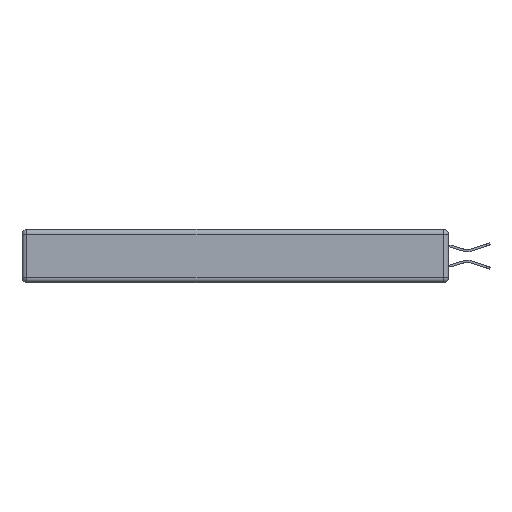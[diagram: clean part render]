
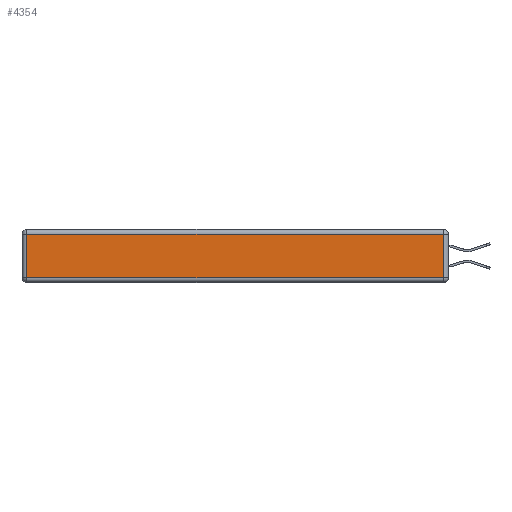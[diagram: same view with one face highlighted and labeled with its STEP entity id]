
A CAD part, left-side view. The second image highlights one B-rep face of the part: STEP entity #4354.
In plain terms, the highlighted planar face has unit normal (-1, 0, 0).
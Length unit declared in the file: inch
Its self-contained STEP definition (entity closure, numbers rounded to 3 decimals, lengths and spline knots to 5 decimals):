
#211 = FACE_OUTER_BOUND ( 'NONE', #3183, .T. ) ;
#361 = VERTEX_POINT ( 'NONE', #15520 ) ;
#588 = VERTEX_POINT ( 'NONE', #12905 ) ;
#858 = LINE ( 'NONE', #8978, #6349 ) ;
#1086 = DIRECTION ( 'NONE',  ( -1., 0., 0. ) ) ;
#1847 = DIRECTION ( 'NONE',  ( 0., 0., -1. ) ) ;
#2959 = AXIS2_PLACEMENT_3D ( 'NONE', #13436, #1086, #5044 ) ;
#3183 = EDGE_LOOP ( 'NONE', ( #13286, #7519, #15727, #15688 ) ) ;
#3670 = EDGE_CURVE ( 'NONE', #4537, #588, #15774, .T. ) ;
#4354 = ADVANCED_FACE ( 'NONE', ( #211 ), #10947, .T. ) ;
#4537 = VERTEX_POINT ( 'NONE', #11445 ) ;
#5044 = DIRECTION ( 'NONE',  ( 0., 0., 1. ) ) ;
#6349 = VECTOR ( 'NONE', #9141, 39.37008 ) ;
#7519 = ORIENTED_EDGE ( 'NONE', *, *, #15940, .T. ) ;
#7658 = EDGE_CURVE ( 'NONE', #361, #4537, #9365, .T. ) ;
#8339 = EDGE_CURVE ( 'NONE', #13849, #361, #8760, .T. ) ;
#8760 = LINE ( 'NONE', #9498, #12446 ) ;
#8972 = VECTOR ( 'NONE', #1847, 39.37008 ) ;
#8978 = CARTESIAN_POINT ( 'NONE',  ( 0., 0.03, -0.343 ) ) ;
#9141 = DIRECTION ( 'NONE',  ( 0., 0., 1. ) ) ;
#9365 = LINE ( 'NONE', #11850, #8972 ) ;
#9498 = CARTESIAN_POINT ( 'NONE',  ( 0., 2.75, -0.03 ) ) ;
#9984 = DIRECTION ( 'NONE',  ( 0., 1., 0. ) ) ;
#10947 = PLANE ( 'NONE',  #2959 ) ;
#11445 = CARTESIAN_POINT ( 'NONE',  ( 0., 2.72, -0.313 ) ) ;
#11850 = CARTESIAN_POINT ( 'NONE',  ( 0., 2.72, -0.343 ) ) ;
#12446 = VECTOR ( 'NONE', #9984, 39.37008 ) ;
#12816 = CARTESIAN_POINT ( 'NONE',  ( 0., 0., -0.313 ) ) ;
#12858 = CARTESIAN_POINT ( 'NONE',  ( 0., 0.03, -0.03 ) ) ;
#12905 = CARTESIAN_POINT ( 'NONE',  ( 0., 0.03, -0.313 ) ) ;
#13286 = ORIENTED_EDGE ( 'NONE', *, *, #3670, .T. ) ;
#13436 = CARTESIAN_POINT ( 'NONE',  ( 0., 0., -0.343 ) ) ;
#13849 = VERTEX_POINT ( 'NONE', #12858 ) ;
#13984 = DIRECTION ( 'NONE',  ( 0., -1., 0. ) ) ;
#14418 = VECTOR ( 'NONE', #13984, 39.37008 ) ;
#15520 = CARTESIAN_POINT ( 'NONE',  ( 0., 2.72, -0.03 ) ) ;
#15688 = ORIENTED_EDGE ( 'NONE', *, *, #7658, .T. ) ;
#15727 = ORIENTED_EDGE ( 'NONE', *, *, #8339, .T. ) ;
#15774 = LINE ( 'NONE', #12816, #14418 ) ;
#15940 = EDGE_CURVE ( 'NONE', #588, #13849, #858, .T. ) ;
